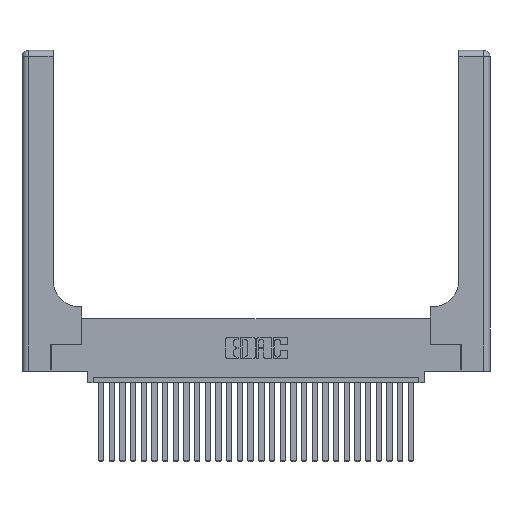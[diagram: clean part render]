
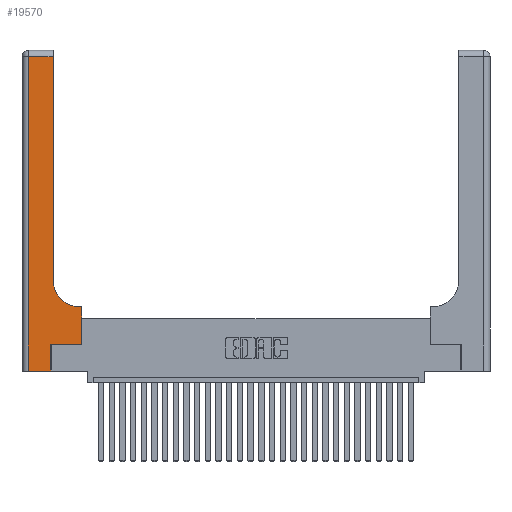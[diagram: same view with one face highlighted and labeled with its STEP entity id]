
A CAD part, top view. The second image highlights one B-rep face of the part: STEP entity #19570.
In plain terms, the highlighted planar face has unit normal (0, 0, 1).
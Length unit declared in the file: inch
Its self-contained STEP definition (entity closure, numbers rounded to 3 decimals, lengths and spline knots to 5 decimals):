
#1170 = DIRECTION ( 'NONE',  ( 0., 0., -1. ) ) ;
#1410 = LINE ( 'NONE', #4019, #17263 ) ;
#1725 = AXIS2_PLACEMENT_3D ( 'NONE', #19807, #10625, #12876 ) ;
#2795 = CIRCLE ( 'NONE', #6200, 0.25 ) ;
#2885 = VERTEX_POINT ( 'NONE', #8984 ) ;
#3570 = CARTESIAN_POINT ( 'NONE',  ( 0.06, 2.94, 0.37 ) ) ;
#4011 = ORIENTED_EDGE ( 'NONE', *, *, #14674, .T. ) ;
#4019 = CARTESIAN_POINT ( 'NONE',  ( 0.269, 0., 0.37 ) ) ;
#4278 = VERTEX_POINT ( 'NONE', #20931 ) ;
#4604 = VECTOR ( 'NONE', #15627, 39.37008 ) ;
#4909 = VERTEX_POINT ( 'NONE', #9784 ) ;
#4950 = EDGE_CURVE ( 'NONE', #18406, #2885, #17506, .T. ) ;
#5035 = VECTOR ( 'NONE', #11247, 39.37008 ) ;
#5501 = VERTEX_POINT ( 'NONE', #3570 ) ;
#5809 = DIRECTION ( 'NONE',  ( 1., 0., 0. ) ) ;
#6200 = AXIS2_PLACEMENT_3D ( 'NONE', #12885, #1170, #19224 ) ;
#6691 = VECTOR ( 'NONE', #5809, 39.37008 ) ;
#6841 = ORIENTED_EDGE ( 'NONE', *, *, #18200, .T. ) ;
#7294 = EDGE_LOOP ( 'NONE', ( #14197, #11431, #17654, #6841, #4011, #8971, #23616, #21482, #11196 ) ) ;
#7406 = VECTOR ( 'NONE', #17847, 39.37008 ) ;
#7796 = CARTESIAN_POINT ( 'NONE',  ( 0.5585, 0.25, 0.37 ) ) ;
#8971 = ORIENTED_EDGE ( 'NONE', *, *, #19724, .T. ) ;
#8984 = CARTESIAN_POINT ( 'NONE',  ( 0.5585, 0.6, 0.37 ) ) ;
#9784 = CARTESIAN_POINT ( 'NONE',  ( 0.5415, 0.6, 0.37 ) ) ;
#10625 = DIRECTION ( 'NONE',  ( 0., 0., -1. ) ) ;
#10785 = VECTOR ( 'NONE', #26442, 39.37008 ) ;
#11196 = ORIENTED_EDGE ( 'NONE', *, *, #27019, .T. ) ;
#11247 = DIRECTION ( 'NONE',  ( 1., 0., 0. ) ) ;
#11431 = ORIENTED_EDGE ( 'NONE', *, *, #27812, .T. ) ;
#12674 = FACE_OUTER_BOUND ( 'NONE', #7294, .T. ) ;
#12876 = DIRECTION ( 'NONE',  ( -1., 0., 0. ) ) ;
#12885 = CARTESIAN_POINT ( 'NONE',  ( 0.5415, 0.85, 0.37 ) ) ;
#13098 = CARTESIAN_POINT ( 'NONE',  ( 0.06, 0., 0.37 ) ) ;
#13146 = CARTESIAN_POINT ( 'NONE',  ( 0.2915, 3., 0.37 ) ) ;
#13355 = CARTESIAN_POINT ( 'NONE',  ( 0.06, 3., 0.37 ) ) ;
#13388 = LINE ( 'NONE', #15563, #7406 ) ;
#13609 = LINE ( 'NONE', #13146, #10785 ) ;
#14197 = ORIENTED_EDGE ( 'NONE', *, *, #22967, .T. ) ;
#14674 = EDGE_CURVE ( 'NONE', #20932, #17515, #1410, .T. ) ;
#14859 = PLANE ( 'NONE',  #1725 ) ;
#15081 = CARTESIAN_POINT ( 'NONE',  ( 0.269, 0., 0.37 ) ) ;
#15563 = CARTESIAN_POINT ( 'NONE',  ( 0.2915, 0.6, 0.37 ) ) ;
#15627 = DIRECTION ( 'NONE',  ( 0., -1., 0. ) ) ;
#16623 = LINE ( 'NONE', #27014, #5035 ) ;
#17263 = VECTOR ( 'NONE', #21996, 39.37008 ) ;
#17506 = LINE ( 'NONE', #7796, #28543 ) ;
#17515 = VERTEX_POINT ( 'NONE', #20417 ) ;
#17628 = VERTEX_POINT ( 'NONE', #13098 ) ;
#17654 = ORIENTED_EDGE ( 'NONE', *, *, #25814, .T. ) ;
#17847 = DIRECTION ( 'NONE',  ( -1., 0., 0. ) ) ;
#18200 = EDGE_CURVE ( 'NONE', #17628, #20932, #16623, .T. ) ;
#18406 = VERTEX_POINT ( 'NONE', #20436 ) ;
#19224 = DIRECTION ( 'NONE',  ( 1., 0., 0. ) ) ;
#19570 = ADVANCED_FACE ( 'NONE', ( #12674 ), #14859, .F. ) ;
#19670 = EDGE_CURVE ( 'NONE', #2885, #4909, #13388, .T. ) ;
#19724 = EDGE_CURVE ( 'NONE', #17515, #18406, #26857, .T. ) ;
#19807 = CARTESIAN_POINT ( 'NONE',  ( 0., 3., 0.37 ) ) ;
#20417 = CARTESIAN_POINT ( 'NONE',  ( 0.269, 0.25, 0.37 ) ) ;
#20436 = CARTESIAN_POINT ( 'NONE',  ( 0.5585, 0.25, 0.37 ) ) ;
#20931 = CARTESIAN_POINT ( 'NONE',  ( 0.2915, 0.85, 0.37 ) ) ;
#20932 = VERTEX_POINT ( 'NONE', #15081 ) ;
#20997 = CARTESIAN_POINT ( 'NONE',  ( 0.269, 0.25, 0.37 ) ) ;
#21144 = VECTOR ( 'NONE', #29217, 39.37008 ) ;
#21482 = ORIENTED_EDGE ( 'NONE', *, *, #19670, .T. ) ;
#21510 = LINE ( 'NONE', #28910, #21144 ) ;
#21996 = DIRECTION ( 'NONE',  ( 0., 1., 0. ) ) ;
#22504 = VERTEX_POINT ( 'NONE', #22581 ) ;
#22581 = CARTESIAN_POINT ( 'NONE',  ( 0.2915, 2.94, 0.37 ) ) ;
#22636 = LINE ( 'NONE', #13355, #4604 ) ;
#22967 = EDGE_CURVE ( 'NONE', #4278, #22504, #13609, .T. ) ;
#23616 = ORIENTED_EDGE ( 'NONE', *, *, #4950, .T. ) ;
#25814 = EDGE_CURVE ( 'NONE', #5501, #17628, #22636, .T. ) ;
#26442 = DIRECTION ( 'NONE',  ( 0., 1., 0. ) ) ;
#26857 = LINE ( 'NONE', #20997, #6691 ) ;
#27014 = CARTESIAN_POINT ( 'NONE',  ( 0., 0., 0.37 ) ) ;
#27019 = EDGE_CURVE ( 'NONE', #4909, #4278, #2795, .T. ) ;
#27791 = DIRECTION ( 'NONE',  ( 0., 1., 0. ) ) ;
#27812 = EDGE_CURVE ( 'NONE', #22504, #5501, #21510, .T. ) ;
#28543 = VECTOR ( 'NONE', #27791, 39.37008 ) ;
#28910 = CARTESIAN_POINT ( 'NONE',  ( 0., 2.94, 0.37 ) ) ;
#29217 = DIRECTION ( 'NONE',  ( -1., 0., 0. ) ) ;
